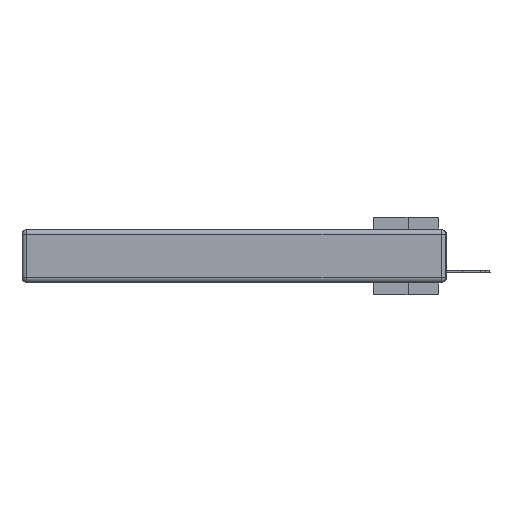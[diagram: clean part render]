
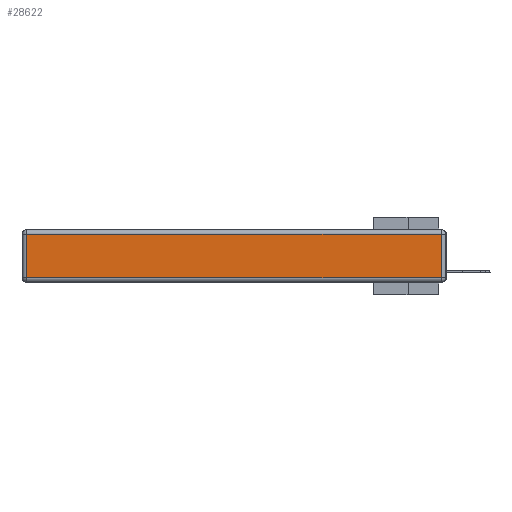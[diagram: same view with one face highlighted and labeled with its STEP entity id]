
A CAD part, left-side view. The second image highlights one B-rep face of the part: STEP entity #28622.
In plain terms, the highlighted planar face has unit normal (-1, 0, 0).
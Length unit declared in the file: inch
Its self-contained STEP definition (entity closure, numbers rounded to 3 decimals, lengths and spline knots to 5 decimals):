
#172 = LINE ( 'NONE', #27077, #25378 ) ;
#195 = EDGE_CURVE ( 'NONE', #7275, #14678, #23842, .T. ) ;
#840 = ORIENTED_EDGE ( 'NONE', *, *, #23330, .T. ) ;
#3265 = VECTOR ( 'NONE', #31596, 39.37008 ) ;
#4113 = PLANE ( 'NONE',  #11942 ) ;
#5699 = DIRECTION ( 'NONE',  ( 0., 1., 0. ) ) ;
#6494 = DIRECTION ( 'NONE',  ( -1., 0., 0. ) ) ;
#6995 = VERTEX_POINT ( 'NONE', #9307 ) ;
#7002 = CARTESIAN_POINT ( 'NONE',  ( 0., 2.72, -0.03 ) ) ;
#7275 = VERTEX_POINT ( 'NONE', #8408 ) ;
#8077 = LINE ( 'NONE', #26766, #12751 ) ;
#8408 = CARTESIAN_POINT ( 'NONE',  ( 0., 2.72, -0.313 ) ) ;
#9174 = EDGE_CURVE ( 'NONE', #14678, #6995, #8077, .T. ) ;
#9307 = CARTESIAN_POINT ( 'NONE',  ( 0., 0.03, -0.03 ) ) ;
#9815 = DIRECTION ( 'NONE',  ( 0., 0., -1. ) ) ;
#11011 = EDGE_LOOP ( 'NONE', ( #31527, #17949, #840, #11621 ) ) ;
#11621 = ORIENTED_EDGE ( 'NONE', *, *, #21439, .T. ) ;
#11942 = AXIS2_PLACEMENT_3D ( 'NONE', #19060, #6494, #31189 ) ;
#12751 = VECTOR ( 'NONE', #16903, 39.37008 ) ;
#14678 = VERTEX_POINT ( 'NONE', #14749 ) ;
#14749 = CARTESIAN_POINT ( 'NONE',  ( 0., 0.03, -0.313 ) ) ;
#16642 = CARTESIAN_POINT ( 'NONE',  ( 0., 0., -0.313 ) ) ;
#16903 = DIRECTION ( 'NONE',  ( 0., 0., 1. ) ) ;
#16973 = VERTEX_POINT ( 'NONE', #7002 ) ;
#17949 = ORIENTED_EDGE ( 'NONE', *, *, #9174, .T. ) ;
#19060 = CARTESIAN_POINT ( 'NONE',  ( 0., 0., -0.343 ) ) ;
#20883 = CARTESIAN_POINT ( 'NONE',  ( 0., 2.75, -0.03 ) ) ;
#21439 = EDGE_CURVE ( 'NONE', #16973, #7275, #172, .T. ) ;
#21552 = FACE_OUTER_BOUND ( 'NONE', #11011, .T. ) ;
#23330 = EDGE_CURVE ( 'NONE', #6995, #16973, #24580, .T. ) ;
#23842 = LINE ( 'NONE', #16642, #3265 ) ;
#24580 = LINE ( 'NONE', #20883, #27275 ) ;
#25378 = VECTOR ( 'NONE', #9815, 39.37008 ) ;
#26766 = CARTESIAN_POINT ( 'NONE',  ( 0., 0.03, -0.343 ) ) ;
#27077 = CARTESIAN_POINT ( 'NONE',  ( 0., 2.72, -0.343 ) ) ;
#27275 = VECTOR ( 'NONE', #5699, 39.37008 ) ;
#28622 = ADVANCED_FACE ( 'NONE', ( #21552 ), #4113, .T. ) ;
#31189 = DIRECTION ( 'NONE',  ( 0., 0., 1. ) ) ;
#31527 = ORIENTED_EDGE ( 'NONE', *, *, #195, .T. ) ;
#31596 = DIRECTION ( 'NONE',  ( 0., -1., 0. ) ) ;
